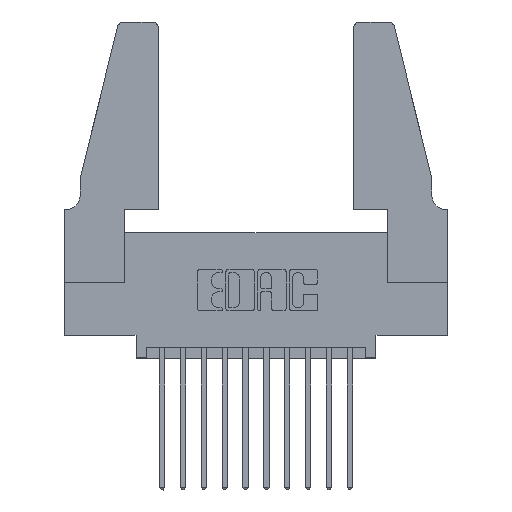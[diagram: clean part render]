
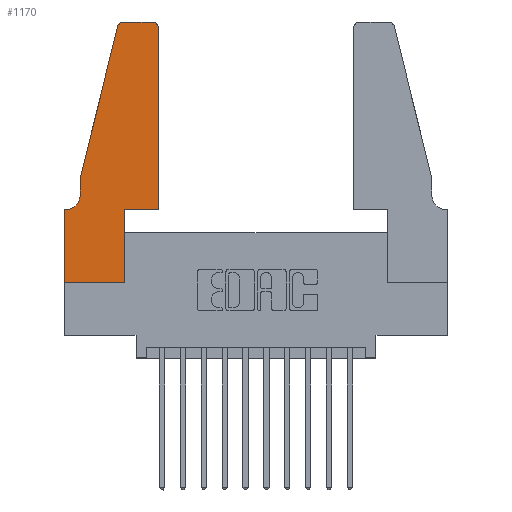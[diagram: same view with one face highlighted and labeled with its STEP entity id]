
A CAD part, top view. The second image highlights one B-rep face of the part: STEP entity #1170.
In plain terms, the highlighted planar face has unit normal (0, 0, 1).
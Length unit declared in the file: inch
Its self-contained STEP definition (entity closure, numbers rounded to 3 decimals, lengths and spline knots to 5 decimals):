
#42 = VERTEX_POINT ( 'NONE', #4998 ) ;
#96 = DIRECTION ( 'NONE',  ( 1., 0., 0. ) ) ;
#359 = EDGE_CURVE ( 'NONE', #7935, #14342, #14375, .T. ) ;
#398 = EDGE_CURVE ( 'NONE', #42, #12639, #14024, .T. ) ;
#781 = ORIENTED_EDGE ( 'NONE', *, *, #359, .T. ) ;
#1170 = ADVANCED_FACE ( 'NONE', ( #6161 ), #12280, .T. ) ;
#1277 = EDGE_CURVE ( 'NONE', #6820, #5735, #1987, .T. ) ;
#1394 = ORIENTED_EDGE ( 'NONE', *, *, #13030, .T. ) ;
#1843 = CARTESIAN_POINT ( 'NONE',  ( 0.4505, 1.22, 0.37 ) ) ;
#1918 = CARTESIAN_POINT ( 'NONE',  ( 0.284, 1.25, 0.37 ) ) ;
#1932 = LINE ( 'NONE', #4846, #7858 ) ;
#1982 = CARTESIAN_POINT ( 'NONE',  ( 0.0755, 0.35, 0.37 ) ) ;
#1987 = LINE ( 'NONE', #2181, #2477 ) ;
#2181 = CARTESIAN_POINT ( 'NONE',  ( 0.0755, 0.5, 0.37 ) ) ;
#2242 = LINE ( 'NONE', #8451, #6954 ) ;
#2295 = EDGE_CURVE ( 'NONE', #6935, #12793, #3181, .T. ) ;
#2319 = AXIS2_PLACEMENT_3D ( 'NONE', #8876, #13357, #7828 ) ;
#2388 = CARTESIAN_POINT ( 'NONE',  ( 0., 0., 0.37 ) ) ;
#2477 = VECTOR ( 'NONE', #11382, 39.37008 ) ;
#2511 = CARTESIAN_POINT ( 'NONE',  ( 0.4505, 0.35, 0.37 ) ) ;
#2553 = DIRECTION ( 'NONE',  ( 0., 0., 1. ) ) ;
#2775 = DIRECTION ( 'NONE',  ( 1., 0., 0. ) ) ;
#2828 = CARTESIAN_POINT ( 'NONE',  ( 0.4505, 0.35, 0.37 ) ) ;
#2864 = AXIS2_PLACEMENT_3D ( 'NONE', #6811, #7904, #3636 ) ;
#3181 = LINE ( 'NONE', #2511, #12245 ) ;
#3209 = CARTESIAN_POINT ( 'NONE',  ( 0.4205, 1.25, 0.37 ) ) ;
#3213 = ORIENTED_EDGE ( 'NONE', *, *, #398, .T. ) ;
#3250 = DIRECTION ( 'NONE',  ( -1., 0., 0. ) ) ;
#3274 = CARTESIAN_POINT ( 'NONE',  ( 0.0755, 0.5, 0.37 ) ) ;
#3279 = VERTEX_POINT ( 'NONE', #4963 ) ;
#3323 = ORIENTED_EDGE ( 'NONE', *, *, #8517, .T. ) ;
#3387 = VERTEX_POINT ( 'NONE', #3209 ) ;
#3636 = DIRECTION ( 'NONE',  ( -1., 0., 0. ) ) ;
#3701 = CARTESIAN_POINT ( 'NONE',  ( 0.2865, 0., 0.37 ) ) ;
#3742 = CARTESIAN_POINT ( 'NONE',  ( 0.284, 1.22, 0.37 ) ) ;
#3972 = EDGE_CURVE ( 'NONE', #8752, #3279, #2242, .T. ) ;
#4160 = EDGE_CURVE ( 'NONE', #3387, #12721, #6261, .T. ) ;
#4439 = EDGE_CURVE ( 'NONE', #12721, #6820, #12204, .T. ) ;
#4453 = ORIENTED_EDGE ( 'NONE', *, *, #4160, .T. ) ;
#4482 = CARTESIAN_POINT ( 'NONE',  ( 0.25487, 1.22718, 0.37 ) ) ;
#4699 = LINE ( 'NONE', #1982, #13755 ) ;
#4794 = AXIS2_PLACEMENT_3D ( 'NONE', #3742, #2553, #9369 ) ;
#4846 = CARTESIAN_POINT ( 'NONE',  ( 0., 0., 0.37 ) ) ;
#4963 = CARTESIAN_POINT ( 'NONE',  ( 0.2865, 0.35, 0.37 ) ) ;
#4998 = CARTESIAN_POINT ( 'NONE',  ( 0., 0.35, 0.37 ) ) ;
#5735 = VERTEX_POINT ( 'NONE', #3274 ) ;
#6161 = FACE_OUTER_BOUND ( 'NONE', #12124, .T. ) ;
#6261 = LINE ( 'NONE', #8912, #10278 ) ;
#6351 = DIRECTION ( 'NONE',  ( 0., 1., 0. ) ) ;
#6546 = ORIENTED_EDGE ( 'NONE', *, *, #1277, .T. ) ;
#6757 = DIRECTION ( 'NONE',  ( 0., 0., 1. ) ) ;
#6811 = CARTESIAN_POINT ( 'NONE',  ( 0.0055, 0.42, 0.37 ) ) ;
#6820 = VERTEX_POINT ( 'NONE', #4482 ) ;
#6935 = VERTEX_POINT ( 'NONE', #11129 ) ;
#6954 = VECTOR ( 'NONE', #6351, 39.37008 ) ;
#7241 = VECTOR ( 'NONE', #2775, 39.37008 ) ;
#7396 = EDGE_CURVE ( 'NONE', #12793, #3387, #7799, .T. ) ;
#7695 = DIRECTION ( 'NONE',  ( 0., -1., 0. ) ) ;
#7721 = EDGE_CURVE ( 'NONE', #3279, #6935, #13028, .T. ) ;
#7799 = CIRCLE ( 'NONE', #8433, 0.03 ) ;
#7820 = ORIENTED_EDGE ( 'NONE', *, *, #11708, .T. ) ;
#7828 = DIRECTION ( 'NONE',  ( 1., 0., 0. ) ) ;
#7858 = VECTOR ( 'NONE', #9487, 39.37008 ) ;
#7904 = DIRECTION ( 'NONE',  ( 0., 0., -1. ) ) ;
#7935 = VERTEX_POINT ( 'NONE', #8306 ) ;
#8050 = VECTOR ( 'NONE', #9046, 39.37008 ) ;
#8306 = CARTESIAN_POINT ( 'NONE',  ( 0.0755, 0.42, 0.37 ) ) ;
#8384 = CARTESIAN_POINT ( 'NONE',  ( 0., 0., 0.37 ) ) ;
#8433 = AXIS2_PLACEMENT_3D ( 'NONE', #14464, #6757, #96 ) ;
#8451 = CARTESIAN_POINT ( 'NONE',  ( 0.2865, 0.35, 0.37 ) ) ;
#8517 = EDGE_CURVE ( 'NONE', #5735, #7935, #12314, .T. ) ;
#8752 = VERTEX_POINT ( 'NONE', #3701 ) ;
#8876 = CARTESIAN_POINT ( 'NONE',  ( 0., 0.35, 0.37 ) ) ;
#8912 = CARTESIAN_POINT ( 'NONE',  ( 0.2605, 1.25, 0.37 ) ) ;
#8913 = ORIENTED_EDGE ( 'NONE', *, *, #7396, .T. ) ;
#8914 = CARTESIAN_POINT ( 'NONE',  ( 0.0055, 0.35, 0.37 ) ) ;
#8958 = DIRECTION ( 'NONE',  ( -1., 0., 0. ) ) ;
#9046 = DIRECTION ( 'NONE',  ( 0., -1., 0. ) ) ;
#9320 = VECTOR ( 'NONE', #7695, 39.37008 ) ;
#9369 = DIRECTION ( 'NONE',  ( 1., 0., 0. ) ) ;
#9487 = DIRECTION ( 'NONE',  ( 1., 0., 0. ) ) ;
#10278 = VECTOR ( 'NONE', #8958, 39.37008 ) ;
#10420 = DIRECTION ( 'NONE',  ( 0., 1., 0. ) ) ;
#11129 = CARTESIAN_POINT ( 'NONE',  ( 0.4505, 0.35, 0.37 ) ) ;
#11382 = DIRECTION ( 'NONE',  ( -0.239, -0.971, 0. ) ) ;
#11708 = EDGE_CURVE ( 'NONE', #12639, #8752, #1932, .T. ) ;
#12124 = EDGE_LOOP ( 'NONE', ( #4453, #13634, #6546, #3323, #781, #1394, #3213, #7820, #12618, #12247, #14160, #8913 ) ) ;
#12204 = CIRCLE ( 'NONE', #4794, 0.03 ) ;
#12245 = VECTOR ( 'NONE', #10420, 39.37008 ) ;
#12247 = ORIENTED_EDGE ( 'NONE', *, *, #7721, .T. ) ;
#12280 = PLANE ( 'NONE',  #2319 ) ;
#12314 = LINE ( 'NONE', #14299, #9320 ) ;
#12618 = ORIENTED_EDGE ( 'NONE', *, *, #3972, .T. ) ;
#12639 = VERTEX_POINT ( 'NONE', #8384 ) ;
#12721 = VERTEX_POINT ( 'NONE', #1918 ) ;
#12793 = VERTEX_POINT ( 'NONE', #1843 ) ;
#13028 = LINE ( 'NONE', #2828, #7241 ) ;
#13030 = EDGE_CURVE ( 'NONE', #14342, #42, #4699, .T. ) ;
#13357 = DIRECTION ( 'NONE',  ( 0., 0., 1. ) ) ;
#13634 = ORIENTED_EDGE ( 'NONE', *, *, #4439, .T. ) ;
#13755 = VECTOR ( 'NONE', #3250, 39.37008 ) ;
#14024 = LINE ( 'NONE', #2388, #8050 ) ;
#14160 = ORIENTED_EDGE ( 'NONE', *, *, #2295, .T. ) ;
#14299 = CARTESIAN_POINT ( 'NONE',  ( 0.0755, 0.5, 0.37 ) ) ;
#14342 = VERTEX_POINT ( 'NONE', #8914 ) ;
#14375 = CIRCLE ( 'NONE', #2864, 0.07 ) ;
#14464 = CARTESIAN_POINT ( 'NONE',  ( 0.4205, 1.22, 0.37 ) ) ;
